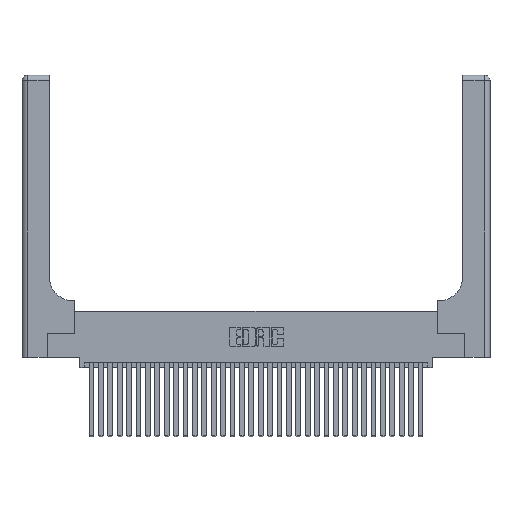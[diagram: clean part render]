
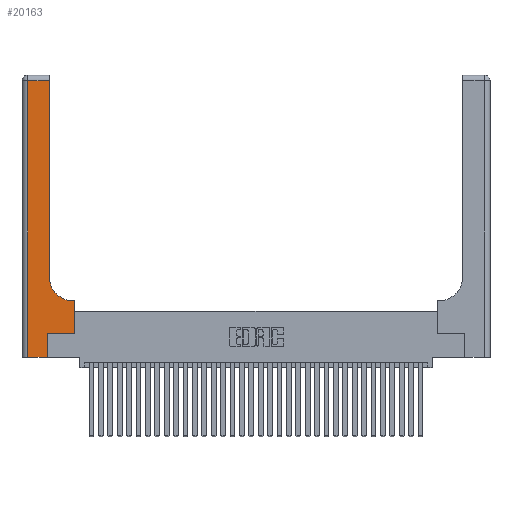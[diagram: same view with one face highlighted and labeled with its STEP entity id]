
A CAD part, top view. The second image highlights one B-rep face of the part: STEP entity #20163.
In plain terms, the highlighted planar face has unit normal (0, 0, 1).
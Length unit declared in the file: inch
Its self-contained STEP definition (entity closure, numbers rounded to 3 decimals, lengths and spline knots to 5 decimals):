
#477 = VERTEX_POINT ( 'NONE', #21502 ) ;
#775 = EDGE_CURVE ( 'NONE', #10053, #5684, #29852, .T. ) ;
#1131 = EDGE_CURVE ( 'NONE', #13554, #11117, #12951, .T. ) ;
#1626 = CARTESIAN_POINT ( 'NONE',  ( 0.269, 0., 0.37 ) ) ;
#1735 = VERTEX_POINT ( 'NONE', #10856 ) ;
#2244 = CARTESIAN_POINT ( 'NONE',  ( 0.06, 3., 0.37 ) ) ;
#2260 = LINE ( 'NONE', #20641, #9354 ) ;
#2625 = LINE ( 'NONE', #1626, #29106 ) ;
#3234 = LINE ( 'NONE', #23305, #24386 ) ;
#4188 = DIRECTION ( 'NONE',  ( 0., 1., 0. ) ) ;
#4744 = DIRECTION ( 'NONE',  ( -1., 0., 0. ) ) ;
#4982 = EDGE_CURVE ( 'NONE', #477, #33196, #3234, .T. ) ;
#5279 = DIRECTION ( 'NONE',  ( 1., 0., 0. ) ) ;
#5684 = VERTEX_POINT ( 'NONE', #26114 ) ;
#5871 = VECTOR ( 'NONE', #29259, 39.37008 ) ;
#5960 = LINE ( 'NONE', #10616, #20100 ) ;
#6779 = CIRCLE ( 'NONE', #21632, 0.25 ) ;
#6853 = EDGE_CURVE ( 'NONE', #5684, #13554, #2260, .T. ) ;
#7297 = DIRECTION ( 'NONE',  ( -1., 0., 0. ) ) ;
#7402 = EDGE_CURVE ( 'NONE', #11117, #1735, #6779, .T. ) ;
#7553 = EDGE_CURVE ( 'NONE', #26322, #10053, #2625, .T. ) ;
#8108 = CARTESIAN_POINT ( 'NONE',  ( 0.2915, 0.6, 0.37 ) ) ;
#8632 = CARTESIAN_POINT ( 'NONE',  ( 0.269, 0.25, 0.37 ) ) ;
#8711 = CARTESIAN_POINT ( 'NONE',  ( 0.06, 2.94, 0.37 ) ) ;
#9014 = LINE ( 'NONE', #12522, #15255 ) ;
#9354 = VECTOR ( 'NONE', #15346, 39.37008 ) ;
#9700 = DIRECTION ( 'NONE',  ( 1., 0., 0. ) ) ;
#10053 = VERTEX_POINT ( 'NONE', #25705 ) ;
#10495 = EDGE_LOOP ( 'NONE', ( #18855, #34002, #20922, #23919, #32502, #19413, #21046, #28004, #23530 ) ) ;
#10616 = CARTESIAN_POINT ( 'NONE',  ( 0., 0., 0.37 ) ) ;
#10856 = CARTESIAN_POINT ( 'NONE',  ( 0.2915, 0.85, 0.37 ) ) ;
#11117 = VERTEX_POINT ( 'NONE', #14013 ) ;
#11848 = LINE ( 'NONE', #2244, #32015 ) ;
#12522 = CARTESIAN_POINT ( 'NONE',  ( 0.2915, 3., 0.37 ) ) ;
#12951 = LINE ( 'NONE', #8108, #5871 ) ;
#13310 = EDGE_CURVE ( 'NONE', #1735, #477, #9014, .T. ) ;
#13554 = VERTEX_POINT ( 'NONE', #21552 ) ;
#14013 = CARTESIAN_POINT ( 'NONE',  ( 0.5415, 0.6, 0.37 ) ) ;
#14475 = CARTESIAN_POINT ( 'NONE',  ( 0.5415, 0.85, 0.37 ) ) ;
#15245 = DIRECTION ( 'NONE',  ( 0., 1., 0. ) ) ;
#15255 = VECTOR ( 'NONE', #15245, 39.37008 ) ;
#15346 = DIRECTION ( 'NONE',  ( 0., 1., 0. ) ) ;
#15659 = AXIS2_PLACEMENT_3D ( 'NONE', #28352, #23224, #7297 ) ;
#16730 = VECTOR ( 'NONE', #9700, 39.37008 ) ;
#17108 = DIRECTION ( 'NONE',  ( 1., 0., 0. ) ) ;
#17929 = PLANE ( 'NONE',  #15659 ) ;
#18855 = ORIENTED_EDGE ( 'NONE', *, *, #13310, .T. ) ;
#19413 = ORIENTED_EDGE ( 'NONE', *, *, #775, .T. ) ;
#20100 = VECTOR ( 'NONE', #5279, 39.37008 ) ;
#20163 = ADVANCED_FACE ( 'NONE', ( #27632 ), #17929, .F. ) ;
#20641 = CARTESIAN_POINT ( 'NONE',  ( 0.5585, 0.25, 0.37 ) ) ;
#20922 = ORIENTED_EDGE ( 'NONE', *, *, #33920, .T. ) ;
#21046 = ORIENTED_EDGE ( 'NONE', *, *, #6853, .T. ) ;
#21502 = CARTESIAN_POINT ( 'NONE',  ( 0.2915, 2.94, 0.37 ) ) ;
#21552 = CARTESIAN_POINT ( 'NONE',  ( 0.5585, 0.6, 0.37 ) ) ;
#21632 = AXIS2_PLACEMENT_3D ( 'NONE', #14475, #32826, #17108 ) ;
#21957 = CARTESIAN_POINT ( 'NONE',  ( 0.06, 0., 0.37 ) ) ;
#22069 = EDGE_CURVE ( 'NONE', #25609, #26322, #5960, .T. ) ;
#23224 = DIRECTION ( 'NONE',  ( 0., 0., -1. ) ) ;
#23305 = CARTESIAN_POINT ( 'NONE',  ( 0., 2.94, 0.37 ) ) ;
#23530 = ORIENTED_EDGE ( 'NONE', *, *, #7402, .T. ) ;
#23919 = ORIENTED_EDGE ( 'NONE', *, *, #22069, .T. ) ;
#24386 = VECTOR ( 'NONE', #4744, 39.37008 ) ;
#25609 = VERTEX_POINT ( 'NONE', #21957 ) ;
#25705 = CARTESIAN_POINT ( 'NONE',  ( 0.269, 0.25, 0.37 ) ) ;
#26114 = CARTESIAN_POINT ( 'NONE',  ( 0.5585, 0.25, 0.37 ) ) ;
#26322 = VERTEX_POINT ( 'NONE', #30593 ) ;
#27632 = FACE_OUTER_BOUND ( 'NONE', #10495, .T. ) ;
#28004 = ORIENTED_EDGE ( 'NONE', *, *, #1131, .T. ) ;
#28352 = CARTESIAN_POINT ( 'NONE',  ( 0., 3., 0.37 ) ) ;
#29106 = VECTOR ( 'NONE', #4188, 39.37008 ) ;
#29259 = DIRECTION ( 'NONE',  ( -1., 0., 0. ) ) ;
#29852 = LINE ( 'NONE', #8632, #16730 ) ;
#30593 = CARTESIAN_POINT ( 'NONE',  ( 0.269, 0., 0.37 ) ) ;
#32015 = VECTOR ( 'NONE', #33848, 39.37008 ) ;
#32502 = ORIENTED_EDGE ( 'NONE', *, *, #7553, .T. ) ;
#32826 = DIRECTION ( 'NONE',  ( 0., 0., -1. ) ) ;
#33196 = VERTEX_POINT ( 'NONE', #8711 ) ;
#33848 = DIRECTION ( 'NONE',  ( 0., -1., 0. ) ) ;
#33920 = EDGE_CURVE ( 'NONE', #33196, #25609, #11848, .T. ) ;
#34002 = ORIENTED_EDGE ( 'NONE', *, *, #4982, .T. ) ;
